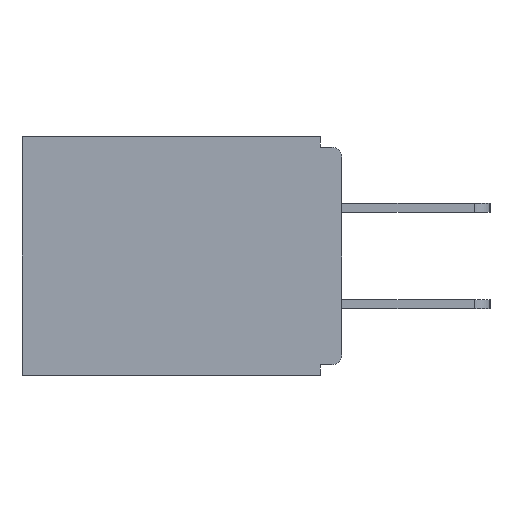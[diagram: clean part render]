
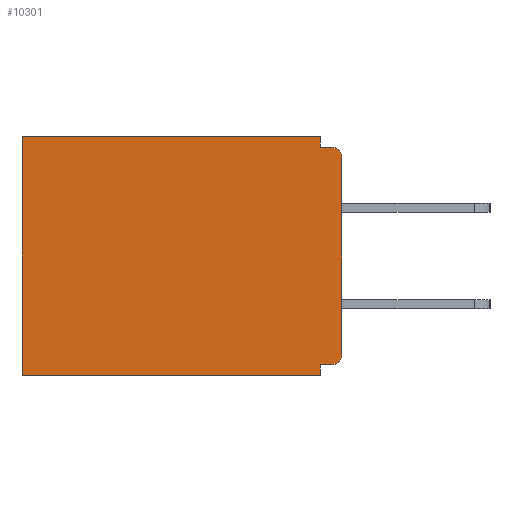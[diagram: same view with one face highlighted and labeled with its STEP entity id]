
A CAD part, left-side view. The second image highlights one B-rep face of the part: STEP entity #10301.
In plain terms, the highlighted planar face has unit normal (-1, 0, 0).
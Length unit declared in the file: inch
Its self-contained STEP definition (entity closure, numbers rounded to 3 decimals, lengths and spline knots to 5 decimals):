
#245 = EDGE_CURVE ( 'NONE', #1803, #16659, #14316, .T. ) ;
#402 = EDGE_CURVE ( 'NONE', #4571, #6884, #15615, .T. ) ;
#434 = VECTOR ( 'NONE', #733, 39.37008 ) ;
#661 = ORIENTED_EDGE ( 'NONE', *, *, #245, .F. ) ;
#733 = DIRECTION ( 'NONE',  ( 0., 0., -1. ) ) ;
#773 = DIRECTION ( 'NONE',  ( 0., 0., -1. ) ) ;
#950 = DIRECTION ( 'NONE',  ( 1., 0., 0. ) ) ;
#979 = VERTEX_POINT ( 'NONE', #14425 ) ;
#1065 = ORIENTED_EDGE ( 'NONE', *, *, #12019, .F. ) ;
#1095 = DIRECTION ( 'NONE',  ( 0., 0., -1. ) ) ;
#1242 = CARTESIAN_POINT ( 'NONE',  ( 0.298, 0.031, 0. ) ) ;
#1580 = CARTESIAN_POINT ( 'NONE',  ( 0.298, 0.031, -0.328 ) ) ;
#1803 = VERTEX_POINT ( 'NONE', #1242 ) ;
#2069 = VECTOR ( 'NONE', #14555, 39.37008 ) ;
#2121 = FACE_OUTER_BOUND ( 'NONE', #14479, .T. ) ;
#2138 = VECTOR ( 'NONE', #1095, 39.37008 ) ;
#2217 = CARTESIAN_POINT ( 'NONE',  ( 0.298, 0.015, -0.328 ) ) ;
#2393 = LINE ( 'NONE', #13224, #434 ) ;
#2770 = VERTEX_POINT ( 'NONE', #15555 ) ;
#3124 = VERTEX_POINT ( 'NONE', #11527 ) ;
#3249 = CIRCLE ( 'NONE', #4852, 0.015 ) ;
#3378 = DIRECTION ( 'NONE',  ( 0., 1., 0. ) ) ;
#3654 = CARTESIAN_POINT ( 'NONE',  ( 0.298, 0., -0.015 ) ) ;
#3706 = CARTESIAN_POINT ( 'NONE',  ( 0.298, 0., -0.313 ) ) ;
#4006 = DIRECTION ( 'NONE',  ( -1., 0., 0. ) ) ;
#4174 = VERTEX_POINT ( 'NONE', #2217 ) ;
#4571 = VERTEX_POINT ( 'NONE', #1580 ) ;
#4852 = AXIS2_PLACEMENT_3D ( 'NONE', #15766, #17154, #10225 ) ;
#5518 = ORIENTED_EDGE ( 'NONE', *, *, #16120, .T. ) ;
#5966 = ORIENTED_EDGE ( 'NONE', *, *, #17160, .F. ) ;
#6004 = CARTESIAN_POINT ( 'NONE',  ( 0.298, 0.031, -0.015 ) ) ;
#6394 = CARTESIAN_POINT ( 'NONE',  ( 0.298, 0.031, -0.343 ) ) ;
#6884 = VERTEX_POINT ( 'NONE', #12548 ) ;
#7249 = CARTESIAN_POINT ( 'NONE',  ( 0.298, 0., -0.343 ) ) ;
#7439 = AXIS2_PLACEMENT_3D ( 'NONE', #15269, #4006, #18152 ) ;
#8926 = EDGE_CURVE ( 'NONE', #979, #13963, #2393, .T. ) ;
#9319 = CARTESIAN_POINT ( 'NONE',  ( 0.298, 0., 0. ) ) ;
#9325 = EDGE_CURVE ( 'NONE', #6884, #3124, #10550, .T. ) ;
#9944 = DIRECTION ( 'NONE',  ( 0., 1., 0. ) ) ;
#10225 = DIRECTION ( 'NONE',  ( 0., 0., -1. ) ) ;
#10301 = ADVANCED_FACE ( 'NONE', ( #2121 ), #13564, .F. ) ;
#10363 = ORIENTED_EDGE ( 'NONE', *, *, #12343, .T. ) ;
#10535 = LINE ( 'NONE', #16455, #2138 ) ;
#10550 = LINE ( 'NONE', #7249, #12043 ) ;
#10640 = DIRECTION ( 'NONE',  ( 0., 0., -1. ) ) ;
#10811 = VECTOR ( 'NONE', #16912, 39.37008 ) ;
#11380 = VECTOR ( 'NONE', #9944, 39.37008 ) ;
#11527 = CARTESIAN_POINT ( 'NONE',  ( 0.298, 0.46, -0.343 ) ) ;
#11892 = VECTOR ( 'NONE', #773, 39.37008 ) ;
#12019 = EDGE_CURVE ( 'NONE', #16659, #2770, #12190, .T. ) ;
#12043 = VECTOR ( 'NONE', #3378, 39.37008 ) ;
#12190 = LINE ( 'NONE', #3654, #12645 ) ;
#12245 = DIRECTION ( 'NONE',  ( 0., -1., 0. ) ) ;
#12343 = EDGE_CURVE ( 'NONE', #1803, #16028, #17668, .T. ) ;
#12548 = CARTESIAN_POINT ( 'NONE',  ( 0.298, 0.031, -0.343 ) ) ;
#12637 = CARTESIAN_POINT ( 'NONE',  ( 0.298, 0.031, -0.343 ) ) ;
#12645 = VECTOR ( 'NONE', #12245, 39.37008 ) ;
#12744 = ORIENTED_EDGE ( 'NONE', *, *, #402, .F. ) ;
#13146 = LINE ( 'NONE', #15610, #11380 ) ;
#13224 = CARTESIAN_POINT ( 'NONE',  ( 0.298, 0., 0. ) ) ;
#13260 = ORIENTED_EDGE ( 'NONE', *, *, #8926, .F. ) ;
#13545 = AXIS2_PLACEMENT_3D ( 'NONE', #9319, #950, #10640 ) ;
#13564 = PLANE ( 'NONE',  #13545 ) ;
#13963 = VERTEX_POINT ( 'NONE', #3706 ) ;
#14316 = LINE ( 'NONE', #12637, #10811 ) ;
#14425 = CARTESIAN_POINT ( 'NONE',  ( 0.298, 0., -0.03 ) ) ;
#14479 = EDGE_LOOP ( 'NONE', ( #15358, #1065, #661, #10363, #5518, #16802, #12744, #5966, #14640, #13260 ) ) ;
#14555 = DIRECTION ( 'NONE',  ( 0., 1., 0. ) ) ;
#14640 = ORIENTED_EDGE ( 'NONE', *, *, #17893, .T. ) ;
#15211 = EDGE_CURVE ( 'NONE', #979, #2770, #17555, .T. ) ;
#15269 = CARTESIAN_POINT ( 'NONE',  ( 0.298, 0.015, -0.03 ) ) ;
#15358 = ORIENTED_EDGE ( 'NONE', *, *, #15211, .T. ) ;
#15555 = CARTESIAN_POINT ( 'NONE',  ( 0.298, 0.015, -0.015 ) ) ;
#15610 = CARTESIAN_POINT ( 'NONE',  ( 0.298, 0., -0.328 ) ) ;
#15615 = LINE ( 'NONE', #6394, #11892 ) ;
#15766 = CARTESIAN_POINT ( 'NONE',  ( 0.298, 0.015, -0.313 ) ) ;
#16028 = VERTEX_POINT ( 'NONE', #16164 ) ;
#16120 = EDGE_CURVE ( 'NONE', #16028, #3124, #10535, .T. ) ;
#16164 = CARTESIAN_POINT ( 'NONE',  ( 0.298, 0.46, 0. ) ) ;
#16455 = CARTESIAN_POINT ( 'NONE',  ( 0.298, 0.46, 0. ) ) ;
#16659 = VERTEX_POINT ( 'NONE', #6004 ) ;
#16802 = ORIENTED_EDGE ( 'NONE', *, *, #9325, .F. ) ;
#16912 = DIRECTION ( 'NONE',  ( 0., 0., -1. ) ) ;
#17154 = DIRECTION ( 'NONE',  ( -1., 0., 0. ) ) ;
#17160 = EDGE_CURVE ( 'NONE', #4174, #4571, #13146, .T. ) ;
#17179 = CARTESIAN_POINT ( 'NONE',  ( 0.298, 0., 0. ) ) ;
#17555 = CIRCLE ( 'NONE', #7439, 0.015 ) ;
#17668 = LINE ( 'NONE', #17179, #2069 ) ;
#17893 = EDGE_CURVE ( 'NONE', #4174, #13963, #3249, .T. ) ;
#18152 = DIRECTION ( 'NONE',  ( 0., 0., -1. ) ) ;
